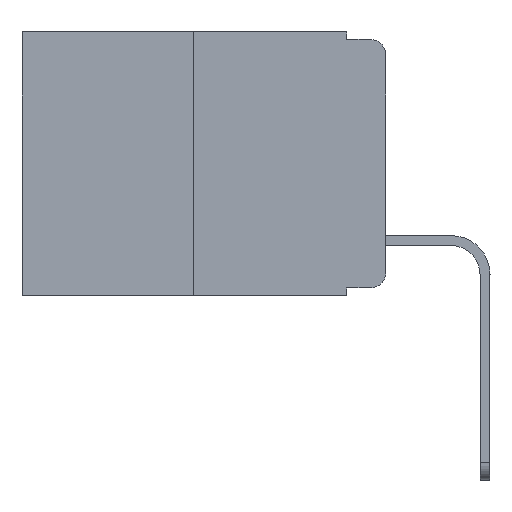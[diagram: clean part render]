
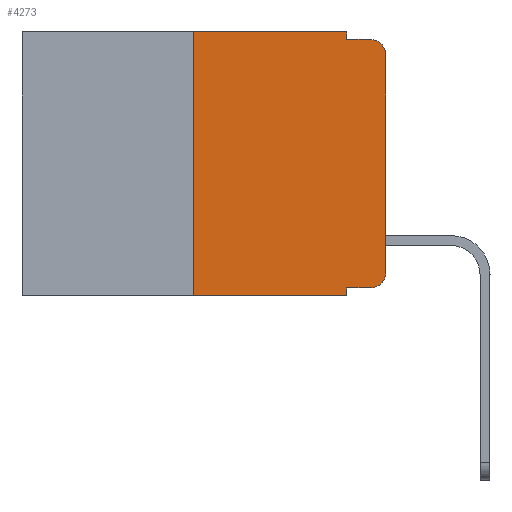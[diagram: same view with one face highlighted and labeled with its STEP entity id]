
A CAD part, left-side view. The second image highlights one B-rep face of the part: STEP entity #4273.
In plain terms, the highlighted planar face has unit normal (-1, 0, 0).
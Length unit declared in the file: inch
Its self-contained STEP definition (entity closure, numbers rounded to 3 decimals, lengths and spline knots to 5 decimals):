
#71 = CARTESIAN_POINT ( 'NONE',  ( 0., 0., -0.03 ) ) ;
#226 = DIRECTION ( 'NONE',  ( 0., 0., -1. ) ) ;
#419 = EDGE_CURVE ( 'NONE', #11310, #5820, #4838, .T. ) ;
#615 = VERTEX_POINT ( 'NONE', #12851 ) ;
#722 = DIRECTION ( 'NONE',  ( 0., -1., 0. ) ) ;
#805 = CARTESIAN_POINT ( 'NONE',  ( 0., 0.02, -0.313 ) ) ;
#1164 = CARTESIAN_POINT ( 'NONE',  ( 0., 0.051, -0.333 ) ) ;
#1285 = CARTESIAN_POINT ( 'NONE',  ( 0., 0.473, 0. ) ) ;
#1465 = DIRECTION ( 'NONE',  ( 0., -1., 0. ) ) ;
#1473 = VERTEX_POINT ( 'NONE', #13238 ) ;
#1544 = CARTESIAN_POINT ( 'NONE',  ( 0., 0., 0. ) ) ;
#1556 = VECTOR ( 'NONE', #1465, 39.37008 ) ;
#1581 = DIRECTION ( 'NONE',  ( 0., 0., 1. ) ) ;
#1860 = CARTESIAN_POINT ( 'NONE',  ( 0., 0.02, -0.333 ) ) ;
#1991 = ORIENTED_EDGE ( 'NONE', *, *, #4024, .T. ) ;
#2128 = LINE ( 'NONE', #14651, #16070 ) ;
#2285 = VERTEX_POINT ( 'NONE', #5993 ) ;
#2343 = DIRECTION ( 'NONE',  ( 0., 0., -1. ) ) ;
#2454 = ORIENTED_EDGE ( 'NONE', *, *, #13667, .F. ) ;
#2783 = EDGE_CURVE ( 'NONE', #15218, #1473, #4800, .T. ) ;
#2965 = EDGE_CURVE ( 'NONE', #6760, #2285, #13619, .T. ) ;
#3362 = AXIS2_PLACEMENT_3D ( 'NONE', #1285, #8126, #226 ) ;
#3544 = ORIENTED_EDGE ( 'NONE', *, *, #9643, .F. ) ;
#3912 = EDGE_CURVE ( 'NONE', #2285, #10808, #11920, .T. ) ;
#4024 = EDGE_CURVE ( 'NONE', #11310, #6760, #4545, .T. ) ;
#4178 = CARTESIAN_POINT ( 'NONE',  ( 0., 0.473, 0. ) ) ;
#4237 = DIRECTION ( 'NONE',  ( 0., 0., -1. ) ) ;
#4273 = ADVANCED_FACE ( 'NONE', ( #9178 ), #9378, .F. ) ;
#4353 = CARTESIAN_POINT ( 'NONE',  ( 0., 0.051, 0. ) ) ;
#4545 = LINE ( 'NONE', #10050, #8127 ) ;
#4690 = CARTESIAN_POINT ( 'NONE',  ( 0., 0.051, 0. ) ) ;
#4800 = LINE ( 'NONE', #4178, #12173 ) ;
#4838 = LINE ( 'NONE', #4690, #11998 ) ;
#5544 = ORIENTED_EDGE ( 'NONE', *, *, #14967, .F. ) ;
#5741 = EDGE_CURVE ( 'NONE', #10808, #6820, #5788, .T. ) ;
#5788 = CIRCLE ( 'NONE', #11413, 0.02 ) ;
#5820 = VERTEX_POINT ( 'NONE', #13764 ) ;
#5993 = CARTESIAN_POINT ( 'NONE',  ( 0., 0., -0.313 ) ) ;
#6141 = VERTEX_POINT ( 'NONE', #7055 ) ;
#6267 = VECTOR ( 'NONE', #4237, 39.37008 ) ;
#6324 = ORIENTED_EDGE ( 'NONE', *, *, #2783, .F. ) ;
#6515 = EDGE_CURVE ( 'NONE', #615, #5820, #2128, .T. ) ;
#6623 = ORIENTED_EDGE ( 'NONE', *, *, #3912, .T. ) ;
#6760 = VERTEX_POINT ( 'NONE', #1860 ) ;
#6820 = VERTEX_POINT ( 'NONE', #12658 ) ;
#7055 = CARTESIAN_POINT ( 'NONE',  ( 0., 0.051, -0.01 ) ) ;
#7090 = LINE ( 'NONE', #13783, #8557 ) ;
#7352 = EDGE_LOOP ( 'NONE', ( #6623, #9088, #3544, #2454, #6324, #5544, #9441, #9581, #1991, #15961 ) ) ;
#7969 = DIRECTION ( 'NONE',  ( 0., -1., 0. ) ) ;
#8126 = DIRECTION ( 'NONE',  ( 1., 0., 0. ) ) ;
#8127 = VECTOR ( 'NONE', #722, 39.37008 ) ;
#8140 = DIRECTION ( 'NONE',  ( 0., -1., 0. ) ) ;
#8557 = VECTOR ( 'NONE', #1581, 39.37008 ) ;
#8858 = DIRECTION ( 'NONE',  ( -1., 0., 0. ) ) ;
#9054 = CARTESIAN_POINT ( 'NONE',  ( 0., 0.02, -0.03 ) ) ;
#9088 = ORIENTED_EDGE ( 'NONE', *, *, #5741, .T. ) ;
#9098 = CARTESIAN_POINT ( 'NONE',  ( 0., 0.25, 0. ) ) ;
#9178 = FACE_OUTER_BOUND ( 'NONE', #7352, .T. ) ;
#9378 = PLANE ( 'NONE',  #3362 ) ;
#9441 = ORIENTED_EDGE ( 'NONE', *, *, #6515, .T. ) ;
#9581 = ORIENTED_EDGE ( 'NONE', *, *, #419, .F. ) ;
#9643 = EDGE_CURVE ( 'NONE', #6141, #6820, #15903, .T. ) ;
#9746 = AXIS2_PLACEMENT_3D ( 'NONE', #805, #8858, #15603 ) ;
#10050 = CARTESIAN_POINT ( 'NONE',  ( 0., 0.051, -0.333 ) ) ;
#10399 = DIRECTION ( 'NONE',  ( -1., 0., 0. ) ) ;
#10732 = CARTESIAN_POINT ( 'NONE',  ( 0., 0.051, -0.01 ) ) ;
#10808 = VERTEX_POINT ( 'NONE', #71 ) ;
#11101 = DIRECTION ( 'NONE',  ( 0., 0., 1. ) ) ;
#11310 = VERTEX_POINT ( 'NONE', #1164 ) ;
#11413 = AXIS2_PLACEMENT_3D ( 'NONE', #9054, #10399, #2343 ) ;
#11702 = VECTOR ( 'NONE', #11101, 39.37008 ) ;
#11920 = LINE ( 'NONE', #1544, #11702 ) ;
#11998 = VECTOR ( 'NONE', #16692, 39.37008 ) ;
#12173 = VECTOR ( 'NONE', #8140, 39.37008 ) ;
#12658 = CARTESIAN_POINT ( 'NONE',  ( 0., 0.02, -0.01 ) ) ;
#12851 = CARTESIAN_POINT ( 'NONE',  ( 0., 0.25, -0.343 ) ) ;
#13238 = CARTESIAN_POINT ( 'NONE',  ( 0., 0.051, 0. ) ) ;
#13619 = CIRCLE ( 'NONE', #9746, 0.02 ) ;
#13667 = EDGE_CURVE ( 'NONE', #1473, #6141, #16579, .T. ) ;
#13764 = CARTESIAN_POINT ( 'NONE',  ( 0., 0.051, -0.343 ) ) ;
#13783 = CARTESIAN_POINT ( 'NONE',  ( 0., 0.25, 0. ) ) ;
#14651 = CARTESIAN_POINT ( 'NONE',  ( 0., 0.473, -0.343 ) ) ;
#14967 = EDGE_CURVE ( 'NONE', #615, #15218, #7090, .T. ) ;
#15218 = VERTEX_POINT ( 'NONE', #9098 ) ;
#15603 = DIRECTION ( 'NONE',  ( 0., 0., -1. ) ) ;
#15903 = LINE ( 'NONE', #10732, #1556 ) ;
#15961 = ORIENTED_EDGE ( 'NONE', *, *, #2965, .T. ) ;
#16070 = VECTOR ( 'NONE', #7969, 39.37008 ) ;
#16579 = LINE ( 'NONE', #4353, #6267 ) ;
#16692 = DIRECTION ( 'NONE',  ( 0., 0., -1. ) ) ;
